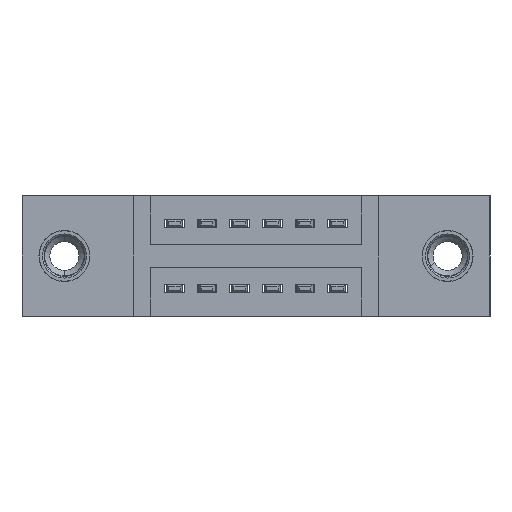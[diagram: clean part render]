
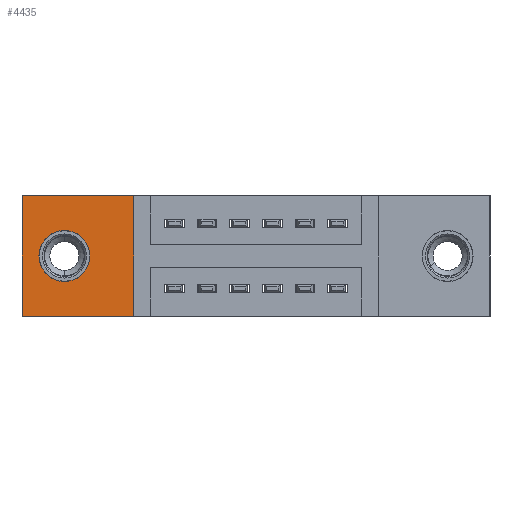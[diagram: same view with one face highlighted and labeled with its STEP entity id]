
A CAD part, front view. The second image highlights one B-rep face of the part: STEP entity #4435.
In plain terms, the highlighted planar face has unit normal (0, -1, 0).
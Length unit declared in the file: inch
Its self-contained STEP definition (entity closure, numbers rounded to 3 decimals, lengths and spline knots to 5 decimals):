
#26 = ORIENTED_EDGE ( 'NONE', *, *, #3457, .F. ) ;
#400 = ORIENTED_EDGE ( 'NONE', *, *, #8043, .F. ) ;
#509 = VERTEX_POINT ( 'NONE', #2165 ) ;
#649 = CIRCLE ( 'NONE', #7292, 0.078 ) ;
#769 = DIRECTION ( 'NONE',  ( 0., -1., 0. ) ) ;
#1104 = EDGE_CURVE ( 'NONE', #5340, #6091, #10109, .T. ) ;
#1212 = LINE ( 'NONE', #7963, #7351 ) ;
#1523 = VERTEX_POINT ( 'NONE', #3764 ) ;
#2011 = VECTOR ( 'NONE', #5983, 39.37008 ) ;
#2165 = CARTESIAN_POINT ( 'NONE',  ( 0.3425, 0.11, -0.37 ) ) ;
#2335 = VERTEX_POINT ( 'NONE', #8292 ) ;
#2351 = EDGE_CURVE ( 'NONE', #6091, #509, #8994, .T. ) ;
#3038 = CARTESIAN_POINT ( 'NONE',  ( 0.13, 0.11, -0.185 ) ) ;
#3114 = EDGE_CURVE ( 'NONE', #2335, #5340, #4261, .T. ) ;
#3457 = EDGE_CURVE ( 'NONE', #7889, #1523, #9566, .T. ) ;
#3653 = EDGE_CURVE ( 'NONE', #509, #2335, #1212, .T. ) ;
#3764 = CARTESIAN_POINT ( 'NONE',  ( 0.13, 0.11, -0.107 ) ) ;
#3807 = CARTESIAN_POINT ( 'NONE',  ( 0., 0.11, 0. ) ) ;
#3886 = DIRECTION ( 'NONE',  ( 0., 0., -1. ) ) ;
#4261 = LINE ( 'NONE', #3807, #2011 ) ;
#4435 = ADVANCED_FACE ( 'NONE', ( #8343, #6182 ), #5819, .T. ) ;
#5061 = ORIENTED_EDGE ( 'NONE', *, *, #3114, .T. ) ;
#5314 = CARTESIAN_POINT ( 'NONE',  ( 0., 0.11, 0. ) ) ;
#5340 = VERTEX_POINT ( 'NONE', #5314 ) ;
#5684 = DIRECTION ( 'NONE',  ( 0., 0., -1. ) ) ;
#5819 = PLANE ( 'NONE',  #9641 ) ;
#5983 = DIRECTION ( 'NONE',  ( -1., 0., 0. ) ) ;
#6091 = VERTEX_POINT ( 'NONE', #9425 ) ;
#6182 = FACE_OUTER_BOUND ( 'NONE', #6784, .T. ) ;
#6656 = DIRECTION ( 'NONE',  ( 0., 0., -1. ) ) ;
#6784 = EDGE_LOOP ( 'NONE', ( #10404, #9732, #8544, #5061 ) ) ;
#6882 = EDGE_LOOP ( 'NONE', ( #400, #26 ) ) ;
#6884 = VECTOR ( 'NONE', #7829, 39.37008 ) ;
#7057 = AXIS2_PLACEMENT_3D ( 'NONE', #10396, #10383, #10379 ) ;
#7292 = AXIS2_PLACEMENT_3D ( 'NONE', #3038, #8795, #3886 ) ;
#7351 = VECTOR ( 'NONE', #9469, 39.37008 ) ;
#7575 = CARTESIAN_POINT ( 'NONE',  ( 0., 0.11, -0.37 ) ) ;
#7829 = DIRECTION ( 'NONE',  ( 1., 0., 0. ) ) ;
#7889 = VERTEX_POINT ( 'NONE', #8630 ) ;
#7963 = CARTESIAN_POINT ( 'NONE',  ( 0.3425, 0.11, 0. ) ) ;
#8043 = EDGE_CURVE ( 'NONE', #1523, #7889, #649, .T. ) ;
#8292 = CARTESIAN_POINT ( 'NONE',  ( 0.3425, 0.11, 0. ) ) ;
#8343 = FACE_BOUND ( 'NONE', #6882, .T. ) ;
#8544 = ORIENTED_EDGE ( 'NONE', *, *, #3653, .T. ) ;
#8576 = CARTESIAN_POINT ( 'NONE',  ( 0., 0.11, 0. ) ) ;
#8630 = CARTESIAN_POINT ( 'NONE',  ( 0.13, 0.11, -0.263 ) ) ;
#8795 = DIRECTION ( 'NONE',  ( 0., -1., 0. ) ) ;
#8994 = LINE ( 'NONE', #7575, #6884 ) ;
#9022 = CARTESIAN_POINT ( 'NONE',  ( 0., 0.11, -0.37 ) ) ;
#9425 = CARTESIAN_POINT ( 'NONE',  ( 0., 0.11, -0.37 ) ) ;
#9469 = DIRECTION ( 'NONE',  ( 0., 0., 1. ) ) ;
#9566 = CIRCLE ( 'NONE', #7057, 0.078 ) ;
#9641 = AXIS2_PLACEMENT_3D ( 'NONE', #9022, #769, #6656 ) ;
#9732 = ORIENTED_EDGE ( 'NONE', *, *, #2351, .T. ) ;
#9871 = VECTOR ( 'NONE', #5684, 39.37008 ) ;
#10109 = LINE ( 'NONE', #8576, #9871 ) ;
#10379 = DIRECTION ( 'NONE',  ( 0., 0., -1. ) ) ;
#10383 = DIRECTION ( 'NONE',  ( 0., -1., 0. ) ) ;
#10396 = CARTESIAN_POINT ( 'NONE',  ( 0.13, 0.11, -0.185 ) ) ;
#10404 = ORIENTED_EDGE ( 'NONE', *, *, #1104, .T. ) ;
